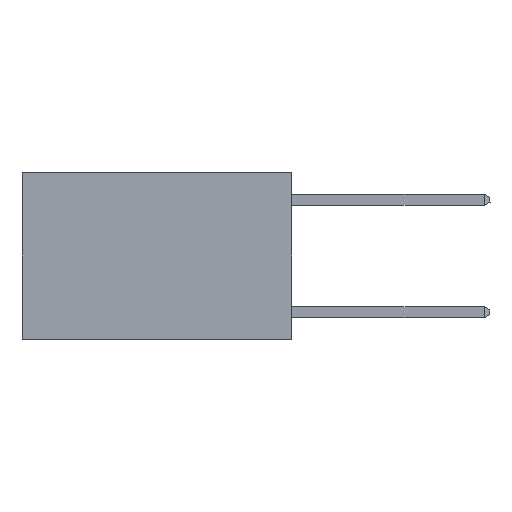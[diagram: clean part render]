
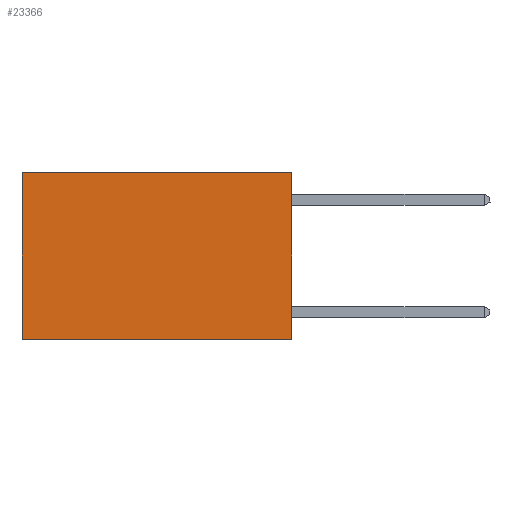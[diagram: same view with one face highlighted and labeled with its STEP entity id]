
A CAD part, left-side view. The second image highlights one B-rep face of the part: STEP entity #23366.
In plain terms, the highlighted planar face has unit normal (-1, 0, 0).
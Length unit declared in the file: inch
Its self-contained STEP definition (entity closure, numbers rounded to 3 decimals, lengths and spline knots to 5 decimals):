
#241 = DIRECTION ( 'NONE',  ( 0., 1., 0. ) ) ;
#252 = EDGE_CURVE ( 'NONE', #5868, #6064, #24909, .T. ) ;
#616 = EDGE_CURVE ( 'NONE', #12594, #6064, #26607, .T. ) ;
#925 = CARTESIAN_POINT ( 'NONE',  ( 0.2625, 0., 0. ) ) ;
#1430 = CARTESIAN_POINT ( 'NONE',  ( 0.2625, 0., 0. ) ) ;
#2534 = VERTEX_POINT ( 'NONE', #1430 ) ;
#4537 = AXIS2_PLACEMENT_3D ( 'NONE', #925, #19140, #5795 ) ;
#5719 = CARTESIAN_POINT ( 'NONE',  ( 0.2625, 0.6, 0. ) ) ;
#5795 = DIRECTION ( 'NONE',  ( 0., 0., -1. ) ) ;
#5868 = VERTEX_POINT ( 'NONE', #12452 ) ;
#6064 = VERTEX_POINT ( 'NONE', #10581 ) ;
#8035 = DIRECTION ( 'NONE',  ( 0., 1., 0. ) ) ;
#8105 = VECTOR ( 'NONE', #20221, 39.37008 ) ;
#10581 = CARTESIAN_POINT ( 'NONE',  ( 0.2625, 0.6, -0.37 ) ) ;
#12452 = CARTESIAN_POINT ( 'NONE',  ( 0.2625, 0.6, 0. ) ) ;
#12594 = VERTEX_POINT ( 'NONE', #22929 ) ;
#13639 = LINE ( 'NONE', #20129, #8105 ) ;
#14981 = ORIENTED_EDGE ( 'NONE', *, *, #616, .F. ) ;
#15745 = CARTESIAN_POINT ( 'NONE',  ( 0.2625, 0., -0.37 ) ) ;
#15753 = CARTESIAN_POINT ( 'NONE',  ( 0.2625, 0., 0. ) ) ;
#16958 = ORIENTED_EDGE ( 'NONE', *, *, #20788, .F. ) ;
#18641 = VECTOR ( 'NONE', #241, 39.37008 ) ;
#19140 = DIRECTION ( 'NONE',  ( 1., 0., 0. ) ) ;
#19390 = LINE ( 'NONE', #15753, #20085 ) ;
#19699 = ORIENTED_EDGE ( 'NONE', *, *, #27458, .T. ) ;
#20085 = VECTOR ( 'NONE', #8035, 39.37008 ) ;
#20129 = CARTESIAN_POINT ( 'NONE',  ( 0.2625, 0., 0. ) ) ;
#20221 = DIRECTION ( 'NONE',  ( 0., 0., -1. ) ) ;
#20788 = EDGE_CURVE ( 'NONE', #2534, #12594, #13639, .T. ) ;
#21914 = ORIENTED_EDGE ( 'NONE', *, *, #252, .T. ) ;
#22929 = CARTESIAN_POINT ( 'NONE',  ( 0.2625, 0., -0.37 ) ) ;
#23248 = FACE_OUTER_BOUND ( 'NONE', #24284, .T. ) ;
#23366 = ADVANCED_FACE ( 'NONE', ( #23248 ), #25925, .F. ) ;
#23812 = DIRECTION ( 'NONE',  ( 0., 0., -1. ) ) ;
#24284 = EDGE_LOOP ( 'NONE', ( #21914, #14981, #16958, #19699 ) ) ;
#24909 = LINE ( 'NONE', #5719, #26271 ) ;
#25925 = PLANE ( 'NONE',  #4537 ) ;
#26271 = VECTOR ( 'NONE', #23812, 39.37008 ) ;
#26607 = LINE ( 'NONE', #15745, #18641 ) ;
#27458 = EDGE_CURVE ( 'NONE', #2534, #5868, #19390, .T. ) ;
